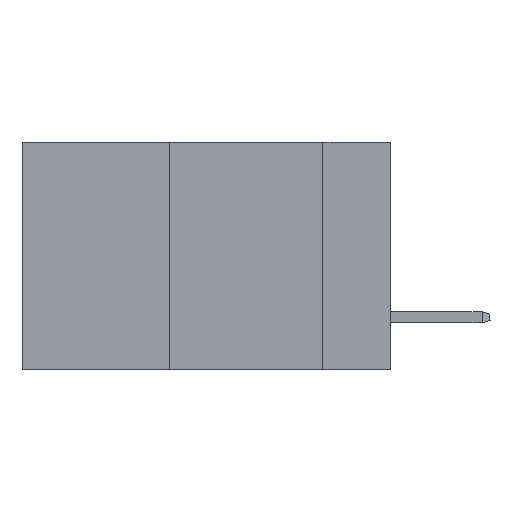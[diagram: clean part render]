
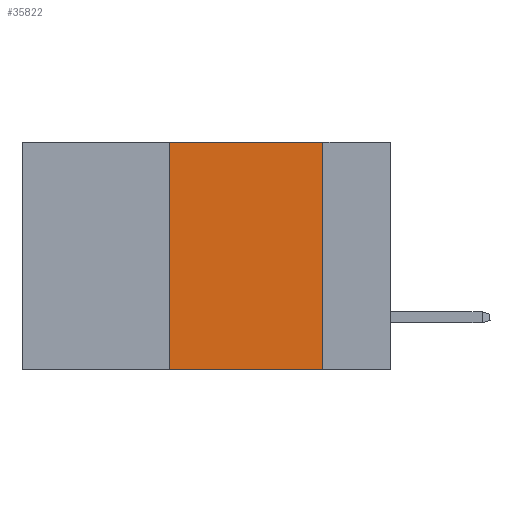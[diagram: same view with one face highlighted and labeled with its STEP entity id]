
A CAD part, left-side view. The second image highlights one B-rep face of the part: STEP entity #35822.
In plain terms, the highlighted planar face has unit normal (-1, 0, 0).
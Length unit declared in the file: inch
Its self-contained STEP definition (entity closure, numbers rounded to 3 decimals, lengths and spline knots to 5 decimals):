
#22 = CARTESIAN_POINT ( 'NONE',  ( 0., 0.11, -0.37 ) ) ;
#356 = CARTESIAN_POINT ( 'NONE',  ( 0., 0.6, 0. ) ) ;
#459 = EDGE_CURVE ( 'NONE', #4798, #1245, #10528, .T. ) ;
#1245 = VERTEX_POINT ( 'NONE', #22 ) ;
#2628 = DIRECTION ( 'NONE',  ( 0., 0., 1. ) ) ;
#4629 = VERTEX_POINT ( 'NONE', #11667 ) ;
#4798 = VERTEX_POINT ( 'NONE', #14984 ) ;
#5360 = LINE ( 'NONE', #21505, #34194 ) ;
#6695 = ORIENTED_EDGE ( 'NONE', *, *, #9934, .F. ) ;
#8461 = DIRECTION ( 'NONE',  ( 0., -1., 0. ) ) ;
#9934 = EDGE_CURVE ( 'NONE', #32273, #4798, #26648, .T. ) ;
#10528 = LINE ( 'NONE', #15136, #33976 ) ;
#11206 = FACE_OUTER_BOUND ( 'NONE', #11795, .T. ) ;
#11667 = CARTESIAN_POINT ( 'NONE',  ( 0., 0.36, -0.37 ) ) ;
#11721 = AXIS2_PLACEMENT_3D ( 'NONE', #356, #35351, #12043 ) ;
#11795 = EDGE_LOOP ( 'NONE', ( #34991, #6695, #37301, #20375 ) ) ;
#12043 = DIRECTION ( 'NONE',  ( 0., 0., -1. ) ) ;
#12285 = PLANE ( 'NONE',  #11721 ) ;
#12340 = VECTOR ( 'NONE', #2628, 39.37008 ) ;
#14585 = EDGE_CURVE ( 'NONE', #4629, #1245, #5360, .T. ) ;
#14984 = CARTESIAN_POINT ( 'NONE',  ( 0., 0.11, 0. ) ) ;
#15136 = CARTESIAN_POINT ( 'NONE',  ( 0., 0.11, 0. ) ) ;
#16852 = CARTESIAN_POINT ( 'NONE',  ( 0., 0.6, 0. ) ) ;
#17248 = VECTOR ( 'NONE', #8461, 39.37008 ) ;
#17488 = EDGE_CURVE ( 'NONE', #4629, #32273, #25422, .T. ) ;
#20375 = ORIENTED_EDGE ( 'NONE', *, *, #14585, .T. ) ;
#20911 = DIRECTION ( 'NONE',  ( 0., 0., -1. ) ) ;
#21505 = CARTESIAN_POINT ( 'NONE',  ( 0., 0.6, -0.37 ) ) ;
#25422 = LINE ( 'NONE', #31802, #12340 ) ;
#26648 = LINE ( 'NONE', #16852, #17248 ) ;
#31802 = CARTESIAN_POINT ( 'NONE',  ( 0., 0.36, 0. ) ) ;
#32273 = VERTEX_POINT ( 'NONE', #33238 ) ;
#33238 = CARTESIAN_POINT ( 'NONE',  ( 0., 0.36, 0. ) ) ;
#33976 = VECTOR ( 'NONE', #20911, 39.37008 ) ;
#34194 = VECTOR ( 'NONE', #35064, 39.37008 ) ;
#34991 = ORIENTED_EDGE ( 'NONE', *, *, #459, .F. ) ;
#35064 = DIRECTION ( 'NONE',  ( 0., -1., 0. ) ) ;
#35351 = DIRECTION ( 'NONE',  ( 1., 0., 0. ) ) ;
#35822 = ADVANCED_FACE ( 'NONE', ( #11206 ), #12285, .F. ) ;
#37301 = ORIENTED_EDGE ( 'NONE', *, *, #17488, .F. ) ;
